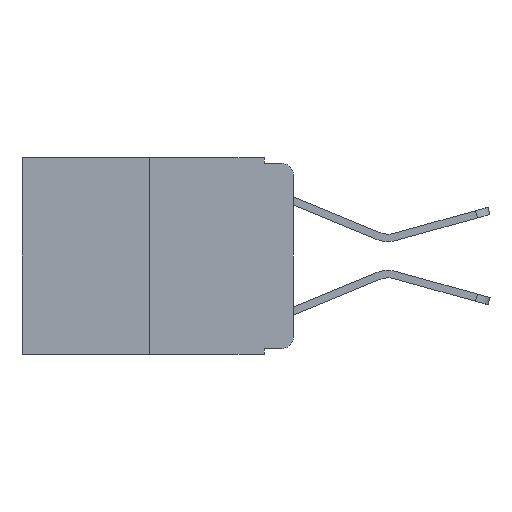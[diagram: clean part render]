
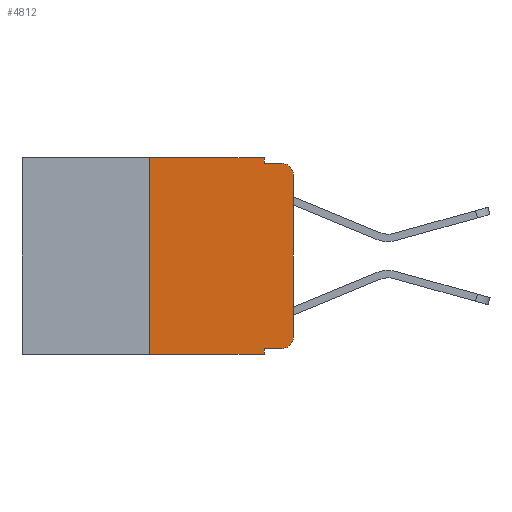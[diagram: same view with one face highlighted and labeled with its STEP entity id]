
A CAD part, left-side view. The second image highlights one B-rep face of the part: STEP entity #4812.
In plain terms, the highlighted planar face has unit normal (-1, 0, 0).
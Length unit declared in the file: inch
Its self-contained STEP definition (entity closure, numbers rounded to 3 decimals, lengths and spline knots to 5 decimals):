
#212 = LINE ( 'NONE', #4433, #12006 ) ;
#227 = VERTEX_POINT ( 'NONE', #9280 ) ;
#370 = LINE ( 'NONE', #10747, #6047 ) ;
#665 = ORIENTED_EDGE ( 'NONE', *, *, #8101, .F. ) ;
#683 = VECTOR ( 'NONE', #2864, 39.37008 ) ;
#843 = EDGE_CURVE ( 'NONE', #6851, #12376, #6071, .T. ) ;
#1001 = PLANE ( 'NONE',  #10915 ) ;
#1073 = DIRECTION ( 'NONE',  ( 0., 0., -1. ) ) ;
#1088 = CARTESIAN_POINT ( 'NONE',  ( 0., 0.051, -0.01 ) ) ;
#1175 = DIRECTION ( 'NONE',  ( 0., 0., -1. ) ) ;
#1386 = VERTEX_POINT ( 'NONE', #8302 ) ;
#1477 = ORIENTED_EDGE ( 'NONE', *, *, #2208, .T. ) ;
#1549 = CARTESIAN_POINT ( 'NONE',  ( 0., 0., -0.03 ) ) ;
#1955 = EDGE_CURVE ( 'NONE', #10595, #4557, #6216, .T. ) ;
#2035 = ORIENTED_EDGE ( 'NONE', *, *, #2122, .F. ) ;
#2122 = EDGE_CURVE ( 'NONE', #4557, #3356, #212, .T. ) ;
#2208 = EDGE_CURVE ( 'NONE', #10707, #6851, #370, .T. ) ;
#2269 = CARTESIAN_POINT ( 'NONE',  ( 0., 0.25, 0. ) ) ;
#2646 = LINE ( 'NONE', #9483, #2983 ) ;
#2864 = DIRECTION ( 'NONE',  ( 0., -1., 0. ) ) ;
#2983 = VECTOR ( 'NONE', #5395, 39.37008 ) ;
#2999 = CARTESIAN_POINT ( 'NONE',  ( 0., 0.02, -0.01 ) ) ;
#3017 = ORIENTED_EDGE ( 'NONE', *, *, #1955, .F. ) ;
#3104 = ORIENTED_EDGE ( 'NONE', *, *, #6615, .T. ) ;
#3189 = CARTESIAN_POINT ( 'NONE',  ( 0., 0.051, 0. ) ) ;
#3212 = DIRECTION ( 'NONE',  ( 0., 0., -1. ) ) ;
#3356 = VERTEX_POINT ( 'NONE', #12592 ) ;
#3624 = ORIENTED_EDGE ( 'NONE', *, *, #8339, .F. ) ;
#3683 = CIRCLE ( 'NONE', #8948, 0.02 ) ;
#4116 = VERTEX_POINT ( 'NONE', #1088 ) ;
#4186 = EDGE_CURVE ( 'NONE', #227, #7010, #6179, .T. ) ;
#4316 = CARTESIAN_POINT ( 'NONE',  ( 0., 0.02, -0.313 ) ) ;
#4433 = CARTESIAN_POINT ( 'NONE',  ( 0., 0.473, 0. ) ) ;
#4557 = VERTEX_POINT ( 'NONE', #2269 ) ;
#4812 = ADVANCED_FACE ( 'NONE', ( #4866 ), #1001, .F. ) ;
#4866 = FACE_OUTER_BOUND ( 'NONE', #8214, .T. ) ;
#5395 = DIRECTION ( 'NONE',  ( 0., -1., 0. ) ) ;
#5497 = DIRECTION ( 'NONE',  ( 0., -1., 0. ) ) ;
#5617 = AXIS2_PLACEMENT_3D ( 'NONE', #13332, #10922, #5757 ) ;
#5757 = DIRECTION ( 'NONE',  ( 0., 0., -1. ) ) ;
#5993 = DIRECTION ( 'NONE',  ( 1., 0., 0. ) ) ;
#6047 = VECTOR ( 'NONE', #12773, 39.37008 ) ;
#6071 = CIRCLE ( 'NONE', #5617, 0.02 ) ;
#6179 = LINE ( 'NONE', #3189, #8429 ) ;
#6216 = LINE ( 'NONE', #9345, #8465 ) ;
#6408 = ORIENTED_EDGE ( 'NONE', *, *, #7856, .T. ) ;
#6615 = EDGE_CURVE ( 'NONE', #1386, #10707, #3683, .T. ) ;
#6715 = ORIENTED_EDGE ( 'NONE', *, *, #843, .T. ) ;
#6851 = VERTEX_POINT ( 'NONE', #1549 ) ;
#7003 = LINE ( 'NONE', #9083, #683 ) ;
#7010 = VERTEX_POINT ( 'NONE', #11933 ) ;
#7505 = CARTESIAN_POINT ( 'NONE',  ( 0., 0.25, -0.343 ) ) ;
#7731 = CARTESIAN_POINT ( 'NONE',  ( 0., 0.051, -0.01 ) ) ;
#7856 = EDGE_CURVE ( 'NONE', #227, #1386, #2646, .T. ) ;
#8101 = EDGE_CURVE ( 'NONE', #4116, #12376, #12655, .T. ) ;
#8214 = EDGE_LOOP ( 'NONE', ( #1477, #6715, #665, #3624, #2035, #3017, #10252, #8645, #6408, #3104 ) ) ;
#8302 = CARTESIAN_POINT ( 'NONE',  ( 0., 0.02, -0.333 ) ) ;
#8339 = EDGE_CURVE ( 'NONE', #3356, #4116, #11519, .T. ) ;
#8429 = VECTOR ( 'NONE', #1175, 39.37008 ) ;
#8465 = VECTOR ( 'NONE', #12420, 39.37008 ) ;
#8645 = ORIENTED_EDGE ( 'NONE', *, *, #4186, .F. ) ;
#8792 = VECTOR ( 'NONE', #1073, 39.37008 ) ;
#8924 = EDGE_CURVE ( 'NONE', #10595, #7010, #7003, .T. ) ;
#8948 = AXIS2_PLACEMENT_3D ( 'NONE', #4316, #10316, #3212 ) ;
#9083 = CARTESIAN_POINT ( 'NONE',  ( 0., 0.473, -0.343 ) ) ;
#9258 = CARTESIAN_POINT ( 'NONE',  ( 0., 0.473, 0. ) ) ;
#9280 = CARTESIAN_POINT ( 'NONE',  ( 0., 0.051, -0.333 ) ) ;
#9345 = CARTESIAN_POINT ( 'NONE',  ( 0., 0.25, 0. ) ) ;
#9483 = CARTESIAN_POINT ( 'NONE',  ( 0., 0.051, -0.333 ) ) ;
#10252 = ORIENTED_EDGE ( 'NONE', *, *, #8924, .T. ) ;
#10273 = CARTESIAN_POINT ( 'NONE',  ( 0., 0.051, 0. ) ) ;
#10316 = DIRECTION ( 'NONE',  ( -1., 0., 0. ) ) ;
#10595 = VERTEX_POINT ( 'NONE', #7505 ) ;
#10633 = CARTESIAN_POINT ( 'NONE',  ( 0., 0., -0.313 ) ) ;
#10707 = VERTEX_POINT ( 'NONE', #10633 ) ;
#10747 = CARTESIAN_POINT ( 'NONE',  ( 0., 0., 0. ) ) ;
#10915 = AXIS2_PLACEMENT_3D ( 'NONE', #9258, #5993, #11209 ) ;
#10922 = DIRECTION ( 'NONE',  ( -1., 0., 0. ) ) ;
#11209 = DIRECTION ( 'NONE',  ( 0., 0., -1. ) ) ;
#11519 = LINE ( 'NONE', #10273, #8792 ) ;
#11533 = VECTOR ( 'NONE', #11864, 39.37008 ) ;
#11864 = DIRECTION ( 'NONE',  ( 0., -1., 0. ) ) ;
#11933 = CARTESIAN_POINT ( 'NONE',  ( 0., 0.051, -0.343 ) ) ;
#12006 = VECTOR ( 'NONE', #5497, 39.37008 ) ;
#12376 = VERTEX_POINT ( 'NONE', #2999 ) ;
#12420 = DIRECTION ( 'NONE',  ( 0., 0., 1. ) ) ;
#12592 = CARTESIAN_POINT ( 'NONE',  ( 0., 0.051, 0. ) ) ;
#12655 = LINE ( 'NONE', #7731, #11533 ) ;
#12773 = DIRECTION ( 'NONE',  ( 0., 0., 1. ) ) ;
#13332 = CARTESIAN_POINT ( 'NONE',  ( 0., 0.02, -0.03 ) ) ;
